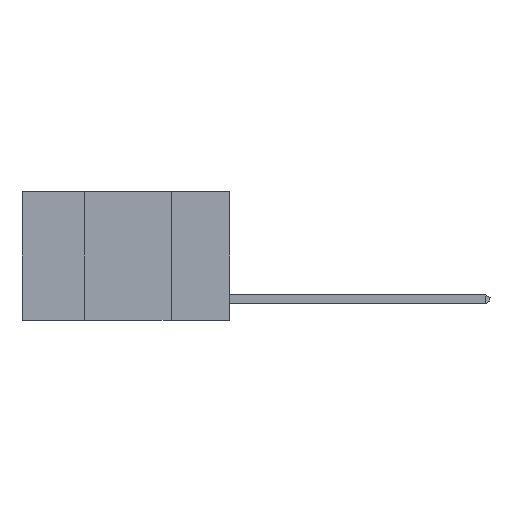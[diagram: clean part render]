
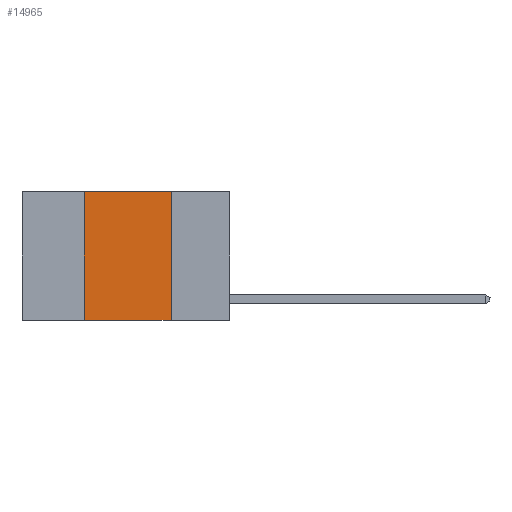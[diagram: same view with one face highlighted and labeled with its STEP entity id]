
A CAD part, left-side view. The second image highlights one B-rep face of the part: STEP entity #14965.
In plain terms, the highlighted planar face has unit normal (-1, 0, 0).
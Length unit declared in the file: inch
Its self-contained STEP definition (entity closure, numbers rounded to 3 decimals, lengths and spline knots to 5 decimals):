
#856 = CARTESIAN_POINT ( 'NONE',  ( 0., 0.42, 0. ) ) ;
#1280 = VECTOR ( 'NONE', #9709, 39.37008 ) ;
#1911 = LINE ( 'NONE', #856, #16064 ) ;
#3365 = CARTESIAN_POINT ( 'NONE',  ( 0., 0.6, -0.37 ) ) ;
#3735 = PLANE ( 'NONE',  #5412 ) ;
#3742 = EDGE_CURVE ( 'NONE', #26949, #13255, #14376, .T. ) ;
#5412 = AXIS2_PLACEMENT_3D ( 'NONE', #19589, #12934, #22145 ) ;
#5998 = EDGE_LOOP ( 'NONE', ( #19889, #23950, #28742, #15358 ) ) ;
#6872 = LINE ( 'NONE', #24690, #22606 ) ;
#6995 = CARTESIAN_POINT ( 'NONE',  ( 0., 0.42, 0. ) ) ;
#8154 = EDGE_CURVE ( 'NONE', #12079, #13255, #13558, .T. ) ;
#9346 = CARTESIAN_POINT ( 'NONE',  ( 0., 0.17, 0. ) ) ;
#9709 = DIRECTION ( 'NONE',  ( 0., -1., 0. ) ) ;
#10056 = EDGE_CURVE ( 'NONE', #26949, #16238, #1911, .T. ) ;
#11419 = CARTESIAN_POINT ( 'NONE',  ( 0., 0.17, -0.37 ) ) ;
#12079 = VERTEX_POINT ( 'NONE', #15924 ) ;
#12934 = DIRECTION ( 'NONE',  ( 1., 0., 0. ) ) ;
#13255 = VERTEX_POINT ( 'NONE', #11419 ) ;
#13558 = LINE ( 'NONE', #9346, #29082 ) ;
#14376 = LINE ( 'NONE', #3365, #1280 ) ;
#14965 = ADVANCED_FACE ( 'NONE', ( #24447 ), #3735, .F. ) ;
#15358 = ORIENTED_EDGE ( 'NONE', *, *, #3742, .T. ) ;
#15924 = CARTESIAN_POINT ( 'NONE',  ( 0., 0.17, 0. ) ) ;
#16064 = VECTOR ( 'NONE', #21504, 39.37008 ) ;
#16238 = VERTEX_POINT ( 'NONE', #6995 ) ;
#19589 = CARTESIAN_POINT ( 'NONE',  ( 0., 0.6, 0. ) ) ;
#19889 = ORIENTED_EDGE ( 'NONE', *, *, #8154, .F. ) ;
#21504 = DIRECTION ( 'NONE',  ( 0., 0., 1. ) ) ;
#21675 = EDGE_CURVE ( 'NONE', #16238, #12079, #6872, .T. ) ;
#21791 = CARTESIAN_POINT ( 'NONE',  ( 0., 0.42, -0.37 ) ) ;
#22145 = DIRECTION ( 'NONE',  ( 0., 0., -1. ) ) ;
#22250 = DIRECTION ( 'NONE',  ( 0., -1., 0. ) ) ;
#22606 = VECTOR ( 'NONE', #22250, 39.37008 ) ;
#23243 = DIRECTION ( 'NONE',  ( 0., 0., -1. ) ) ;
#23950 = ORIENTED_EDGE ( 'NONE', *, *, #21675, .F. ) ;
#24447 = FACE_OUTER_BOUND ( 'NONE', #5998, .T. ) ;
#24690 = CARTESIAN_POINT ( 'NONE',  ( 0., 0.6, 0. ) ) ;
#26949 = VERTEX_POINT ( 'NONE', #21791 ) ;
#28742 = ORIENTED_EDGE ( 'NONE', *, *, #10056, .F. ) ;
#29082 = VECTOR ( 'NONE', #23243, 39.37008 ) ;
